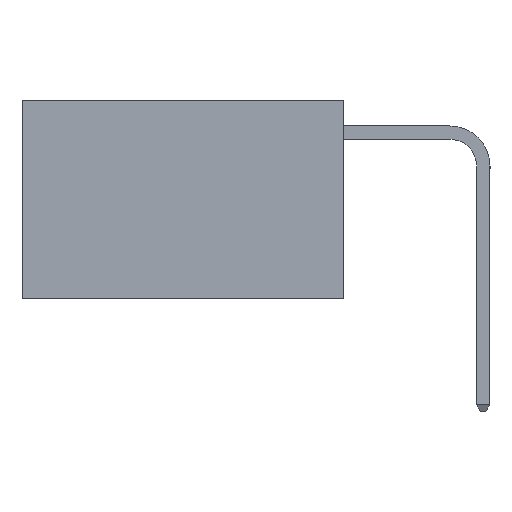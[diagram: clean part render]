
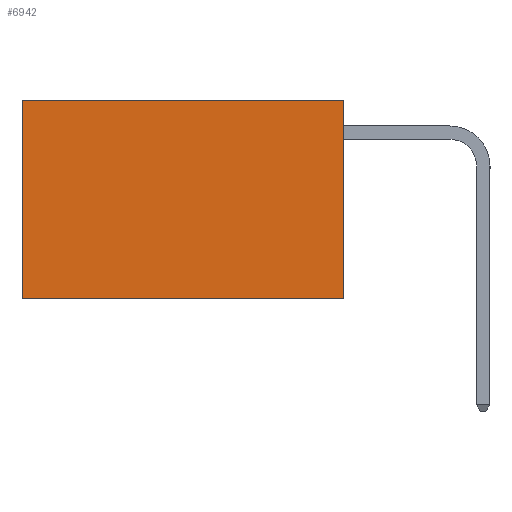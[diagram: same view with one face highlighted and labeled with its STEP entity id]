
A CAD part, left-side view. The second image highlights one B-rep face of the part: STEP entity #6942.
In plain terms, the highlighted planar face has unit normal (-1, 0, 0).
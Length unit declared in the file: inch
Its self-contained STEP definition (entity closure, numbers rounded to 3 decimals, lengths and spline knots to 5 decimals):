
#2102 = VERTEX_POINT ( 'NONE', #2745 ) ;
#2131 = VECTOR ( 'NONE', #13852, 39.37008 ) ;
#2647 = LINE ( 'NONE', #12271, #2131 ) ;
#2745 = CARTESIAN_POINT ( 'NONE',  ( 0.2625, 0.6, 0. ) ) ;
#3653 = VECTOR ( 'NONE', #5487, 39.37008 ) ;
#3851 = CARTESIAN_POINT ( 'NONE',  ( 0.2625, 0., 0. ) ) ;
#5298 = CARTESIAN_POINT ( 'NONE',  ( 0.2625, 0.6, -0.37 ) ) ;
#5487 = DIRECTION ( 'NONE',  ( 0., 0., -1. ) ) ;
#5497 = EDGE_CURVE ( 'NONE', #14263, #8335, #16797, .T. ) ;
#5885 = FACE_OUTER_BOUND ( 'NONE', #5945, .T. ) ;
#5945 = EDGE_LOOP ( 'NONE', ( #11994, #10817, #12770, #14536 ) ) ;
#6663 = CARTESIAN_POINT ( 'NONE',  ( 0.2625, 0., -0.37 ) ) ;
#6942 = ADVANCED_FACE ( 'NONE', ( #5885 ), #13717, .F. ) ;
#7960 = VECTOR ( 'NONE', #15067, 39.37008 ) ;
#8335 = VERTEX_POINT ( 'NONE', #6663 ) ;
#8515 = LINE ( 'NONE', #19600, #12218 ) ;
#8979 = CARTESIAN_POINT ( 'NONE',  ( 0.2625, 0., 0. ) ) ;
#9045 = DIRECTION ( 'NONE',  ( 0., 0., -1. ) ) ;
#10002 = EDGE_CURVE ( 'NONE', #14263, #2102, #2647, .T. ) ;
#10817 = ORIENTED_EDGE ( 'NONE', *, *, #16711, .F. ) ;
#11836 = VERTEX_POINT ( 'NONE', #5298 ) ;
#11994 = ORIENTED_EDGE ( 'NONE', *, *, #17867, .T. ) ;
#12218 = VECTOR ( 'NONE', #13423, 39.37008 ) ;
#12271 = CARTESIAN_POINT ( 'NONE',  ( 0.2625, 0., 0. ) ) ;
#12770 = ORIENTED_EDGE ( 'NONE', *, *, #5497, .F. ) ;
#13423 = DIRECTION ( 'NONE',  ( 0., 1., 0. ) ) ;
#13717 = PLANE ( 'NONE',  #20515 ) ;
#13852 = DIRECTION ( 'NONE',  ( 0., 1., 0. ) ) ;
#14263 = VERTEX_POINT ( 'NONE', #3851 ) ;
#14536 = ORIENTED_EDGE ( 'NONE', *, *, #10002, .T. ) ;
#14964 = CARTESIAN_POINT ( 'NONE',  ( 0.2625, 0.6, 0. ) ) ;
#15067 = DIRECTION ( 'NONE',  ( 0., 0., -1. ) ) ;
#15838 = LINE ( 'NONE', #14964, #3653 ) ;
#16711 = EDGE_CURVE ( 'NONE', #8335, #11836, #8515, .T. ) ;
#16797 = LINE ( 'NONE', #18170, #7960 ) ;
#17867 = EDGE_CURVE ( 'NONE', #2102, #11836, #15838, .T. ) ;
#18170 = CARTESIAN_POINT ( 'NONE',  ( 0.2625, 0., 0. ) ) ;
#18396 = DIRECTION ( 'NONE',  ( 1., 0., 0. ) ) ;
#19600 = CARTESIAN_POINT ( 'NONE',  ( 0.2625, 0., -0.37 ) ) ;
#20515 = AXIS2_PLACEMENT_3D ( 'NONE', #8979, #18396, #9045 ) ;
